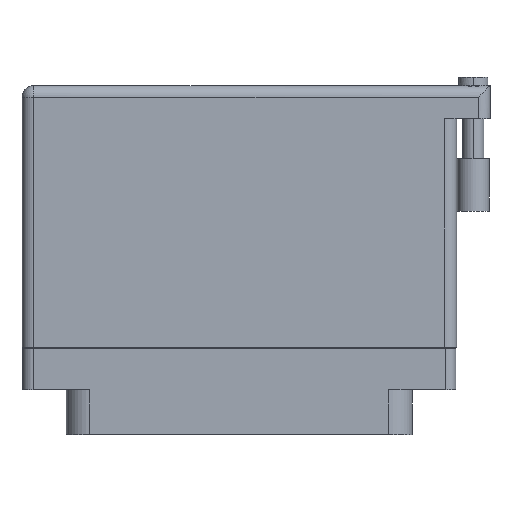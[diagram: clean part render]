
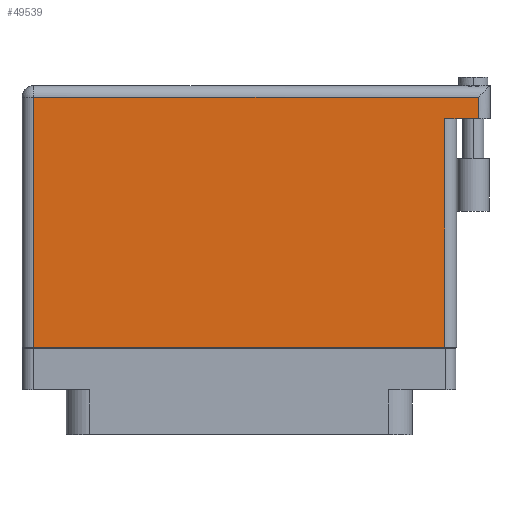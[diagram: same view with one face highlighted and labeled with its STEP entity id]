
A CAD part, front view. The second image highlights one B-rep face of the part: STEP entity #49539.
In plain terms, the highlighted face is planar.
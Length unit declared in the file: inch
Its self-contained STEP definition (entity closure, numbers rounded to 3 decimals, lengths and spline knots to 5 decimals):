
#851 = EDGE_CURVE ( 'NONE', #6685, #44986, #13490, .T. ) ;
#4416 = DIRECTION ( 'NONE',  ( 0., -1., 0. ) ) ;
#4427 = DIRECTION ( 'NONE',  ( 1., 0., 0. ) ) ;
#5661 = ORIENTED_EDGE ( 'NONE', *, *, #49121, .F. ) ;
#6234 = EDGE_LOOP ( 'NONE', ( #21315, #29020, #5661, #43991, #49577, #30244 ) ) ;
#6480 = VECTOR ( 'NONE', #46408, 39.37008 ) ;
#6685 = VERTEX_POINT ( 'NONE', #35212 ) ;
#7983 = EDGE_CURVE ( 'NONE', #15714, #31467, #42402, .T. ) ;
#8758 = DIRECTION ( 'NONE',  ( -1., 0., 0. ) ) ;
#9526 = FACE_OUTER_BOUND ( 'NONE', #6234, .T. ) ;
#10618 = CARTESIAN_POINT ( 'NONE',  ( 1.43, 1.466, 0.4495 ) ) ;
#10637 = CARTESIAN_POINT ( 'NONE',  ( -1.23, -0.1, 0.4495 ) ) ;
#11312 = CARTESIAN_POINT ( 'NONE',  ( 1.23, -0.1, 0.4495 ) ) ;
#12100 = VERTEX_POINT ( 'NONE', #11312 ) ;
#13490 = LINE ( 'NONE', #10618, #50266 ) ;
#13922 = EDGE_CURVE ( 'NONE', #31467, #12100, #39999, .T. ) ;
#14805 = LINE ( 'NONE', #33618, #35367 ) ;
#15714 = VERTEX_POINT ( 'NONE', #40052 ) ;
#16670 = VECTOR ( 'NONE', #20497, 39.37008 ) ;
#16928 = PLANE ( 'NONE',  #30567 ) ;
#17622 = VERTEX_POINT ( 'NONE', #47020 ) ;
#17658 = LINE ( 'NONE', #30304, #6480 ) ;
#19125 = LINE ( 'NONE', #24657, #16670 ) ;
#20497 = DIRECTION ( 'NONE',  ( -1., 0., 0. ) ) ;
#21188 = VECTOR ( 'NONE', #4416, 39.37008 ) ;
#21315 = ORIENTED_EDGE ( 'NONE', *, *, #13922, .T. ) ;
#21965 = EDGE_CURVE ( 'NONE', #12100, #17622, #14805, .T. ) ;
#24017 = CARTESIAN_POINT ( 'NONE',  ( -1.3, -0.1, 0.4495 ) ) ;
#24657 = CARTESIAN_POINT ( 'NONE',  ( -1.3, 1.396, 0.4495 ) ) ;
#26461 = DIRECTION ( 'NONE',  ( 0., 1., 0. ) ) ;
#29020 = ORIENTED_EDGE ( 'NONE', *, *, #21965, .T. ) ;
#30244 = ORIENTED_EDGE ( 'NONE', *, *, #7983, .T. ) ;
#30304 = CARTESIAN_POINT ( 'NONE',  ( 1.5, 1.269, 0.4495 ) ) ;
#30567 = AXIS2_PLACEMENT_3D ( 'NONE', #44809, #32904, #8758 ) ;
#31467 = VERTEX_POINT ( 'NONE', #10637 ) ;
#32904 = DIRECTION ( 'NONE',  ( 0., 0., -1. ) ) ;
#33618 = CARTESIAN_POINT ( 'NONE',  ( 1.23, 1.269, 0.4495 ) ) ;
#35212 = CARTESIAN_POINT ( 'NONE',  ( 1.43, 1.269, 0.4495 ) ) ;
#35367 = VECTOR ( 'NONE', #45351, 39.37008 ) ;
#38756 = EDGE_CURVE ( 'NONE', #44986, #15714, #19125, .T. ) ;
#39999 = LINE ( 'NONE', #24017, #45032 ) ;
#40050 = CARTESIAN_POINT ( 'NONE',  ( -1.23, -0.1, 0.4495 ) ) ;
#40052 = CARTESIAN_POINT ( 'NONE',  ( -1.23, 1.396, 0.4495 ) ) ;
#42402 = LINE ( 'NONE', #40050, #21188 ) ;
#43991 = ORIENTED_EDGE ( 'NONE', *, *, #851, .T. ) ;
#44809 = CARTESIAN_POINT ( 'NONE',  ( -1.3, 1.466, 0.4495 ) ) ;
#44986 = VERTEX_POINT ( 'NONE', #45250 ) ;
#45032 = VECTOR ( 'NONE', #4427, 39.37008 ) ;
#45250 = CARTESIAN_POINT ( 'NONE',  ( 1.43, 1.396, 0.4495 ) ) ;
#45351 = DIRECTION ( 'NONE',  ( 0., 1., 0. ) ) ;
#46408 = DIRECTION ( 'NONE',  ( -1., 0., 0. ) ) ;
#47020 = CARTESIAN_POINT ( 'NONE',  ( 1.23, 1.269, 0.4495 ) ) ;
#49121 = EDGE_CURVE ( 'NONE', #6685, #17622, #17658, .T. ) ;
#49539 = ADVANCED_FACE ( 'NONE', ( #9526 ), #16928, .F. ) ;
#49577 = ORIENTED_EDGE ( 'NONE', *, *, #38756, .T. ) ;
#50266 = VECTOR ( 'NONE', #26461, 39.37008 ) ;
